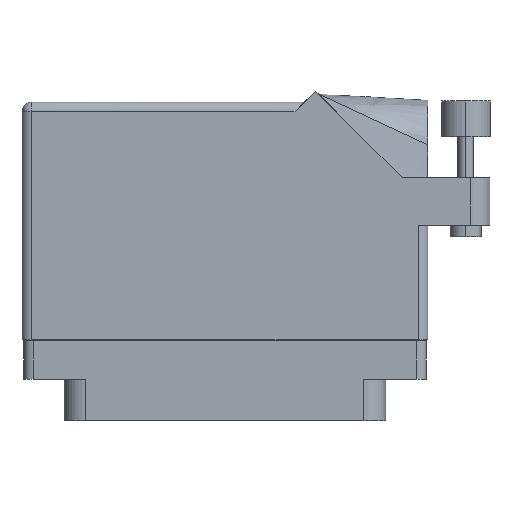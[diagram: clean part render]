
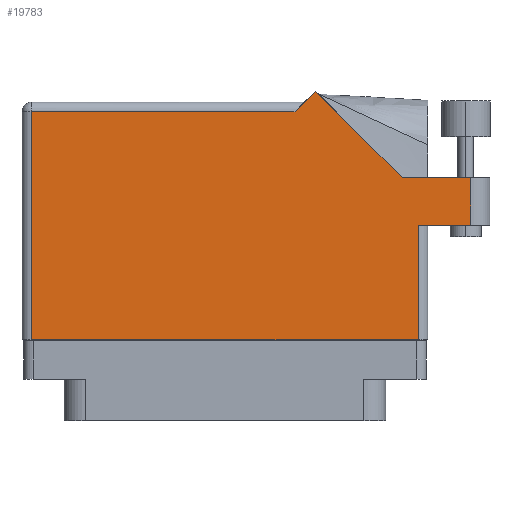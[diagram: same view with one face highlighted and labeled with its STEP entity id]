
A CAD part, front view. The second image highlights one B-rep face of the part: STEP entity #19783.
In plain terms, the highlighted face is planar.
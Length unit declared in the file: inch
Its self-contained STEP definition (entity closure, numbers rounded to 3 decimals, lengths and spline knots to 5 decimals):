
#67 = DIRECTION ( 'NONE',  ( 1., 0., 0. ) ) ;
#538 = LINE ( 'NONE', #2340, #21305 ) ;
#660 = DIRECTION ( 'NONE',  ( -1., 0., 0. ) ) ;
#719 = LINE ( 'NONE', #8086, #8934 ) ;
#1212 = CARTESIAN_POINT ( 'NONE',  ( -1.306, -0.1, 0.455 ) ) ;
#2261 = VERTEX_POINT ( 'NONE', #24734 ) ;
#2340 = CARTESIAN_POINT ( 'NONE',  ( -1.244, -0.1, 0.455 ) ) ;
#3207 = ORIENTED_EDGE ( 'NONE', *, *, #8505, .T. ) ;
#4813 = DIRECTION ( 'NONE',  ( 0., 1., 0. ) ) ;
#5505 = ORIENTED_EDGE ( 'NONE', *, *, #15863, .T. ) ;
#6879 = LINE ( 'NONE', #20447, #30777 ) ;
#7275 = CARTESIAN_POINT ( 'NONE',  ( -1.244, -0.1, 0.455 ) ) ;
#7640 = DIRECTION ( 'NONE',  ( -1., 0., 0. ) ) ;
#8086 = CARTESIAN_POINT ( 'NONE',  ( 1.244, 0.637, 0.455 ) ) ;
#8190 = CARTESIAN_POINT ( 'NONE',  ( 1.306, 0.637, 0.455 ) ) ;
#8468 = CARTESIAN_POINT ( 'NONE',  ( 1.244, 0.637, 0.455 ) ) ;
#8501 = ORIENTED_EDGE ( 'NONE', *, *, #39353, .T. ) ;
#8505 = EDGE_CURVE ( 'NONE', #20362, #31345, #9604, .T. ) ;
#8934 = VECTOR ( 'NONE', #16017, 39.37008 ) ;
#9604 = LINE ( 'NONE', #16311, #18359 ) ;
#9790 = VERTEX_POINT ( 'NONE', #28923 ) ;
#10340 = DIRECTION ( 'NONE',  ( 0., -1., 0. ) ) ;
#10912 = VECTOR ( 'NONE', #50028, 39.37008 ) ;
#11118 = LINE ( 'NONE', #38775, #38047 ) ;
#12791 = EDGE_CURVE ( 'NONE', #9790, #2261, #25380, .T. ) ;
#13012 = CARTESIAN_POINT ( 'NONE',  ( 1.581, 0.637, 0.455 ) ) ;
#13116 = VERTEX_POINT ( 'NONE', #32219 ) ;
#13399 = VECTOR ( 'NONE', #7640, 39.37008 ) ;
#15828 = VECTOR ( 'NONE', #25797, 39.37008 ) ;
#15863 = EDGE_CURVE ( 'NONE', #13116, #21442, #719, .T. ) ;
#16017 = DIRECTION ( 'NONE',  ( 0., 1., 0. ) ) ;
#16311 = CARTESIAN_POINT ( 'NONE',  ( 1.706, 0.944, 0.455 ) ) ;
#16802 = ORIENTED_EDGE ( 'NONE', *, *, #24436, .T. ) ;
#16983 = VECTOR ( 'NONE', #67, 39.37008 ) ;
#18359 = VECTOR ( 'NONE', #48630, 39.37008 ) ;
#18915 = VERTEX_POINT ( 'NONE', #35997 ) ;
#19783 = ADVANCED_FACE ( 'NONE', ( #29522 ), #24737, .F. ) ;
#20362 = VERTEX_POINT ( 'NONE', #50252 ) ;
#20447 = CARTESIAN_POINT ( 'NONE',  ( 1.581, 0.944, 0.455 ) ) ;
#20594 = CARTESIAN_POINT ( 'NONE',  ( 1.14042, 0.944, 0.455 ) ) ;
#20630 = EDGE_CURVE ( 'NONE', #18915, #27556, #538, .T. ) ;
#21305 = VECTOR ( 'NONE', #10340, 39.37008 ) ;
#21442 = VERTEX_POINT ( 'NONE', #8468 ) ;
#22041 = ORIENTED_EDGE ( 'NONE', *, *, #23188, .T. ) ;
#23025 = EDGE_CURVE ( 'NONE', #44366, #20362, #6879, .T. ) ;
#23188 = EDGE_CURVE ( 'NONE', #21442, #44366, #49463, .T. ) ;
#24081 = LINE ( 'NONE', #51544, #13399 ) ;
#24436 = EDGE_CURVE ( 'NONE', #31345, #9790, #11118, .T. ) ;
#24734 = CARTESIAN_POINT ( 'NONE',  ( 0.451, 1.368, 0.455 ) ) ;
#24737 = PLANE ( 'NONE',  #29814 ) ;
#25380 = LINE ( 'NONE', #49537, #10912 ) ;
#25797 = DIRECTION ( 'NONE',  ( 1., 0., 0. ) ) ;
#27556 = VERTEX_POINT ( 'NONE', #7275 ) ;
#28923 = CARTESIAN_POINT ( 'NONE',  ( 0.58371, 1.50071, 0.455 ) ) ;
#29522 = FACE_OUTER_BOUND ( 'NONE', #39858, .T. ) ;
#29814 = AXIS2_PLACEMENT_3D ( 'NONE', #40625, #32978, #660 ) ;
#30777 = VECTOR ( 'NONE', #4813, 39.37008 ) ;
#31345 = VERTEX_POINT ( 'NONE', #20594 ) ;
#32219 = CARTESIAN_POINT ( 'NONE',  ( 1.244, -0.1, 0.455 ) ) ;
#32978 = DIRECTION ( 'NONE',  ( 0., 0., -1. ) ) ;
#35997 = CARTESIAN_POINT ( 'NONE',  ( -1.244, 1.368, 0.455 ) ) ;
#36093 = EDGE_CURVE ( 'NONE', #27556, #13116, #47681, .T. ) ;
#38047 = VECTOR ( 'NONE', #47299, 39.37008 ) ;
#38775 = CARTESIAN_POINT ( 'NONE',  ( 1.14042, 0.944, 0.455 ) ) ;
#39070 = ORIENTED_EDGE ( 'NONE', *, *, #12791, .T. ) ;
#39353 = EDGE_CURVE ( 'NONE', #2261, #18915, #24081, .T. ) ;
#39858 = EDGE_LOOP ( 'NONE', ( #22041, #40624, #3207, #16802, #39070, #8501, #47857, #42623, #5505 ) ) ;
#40624 = ORIENTED_EDGE ( 'NONE', *, *, #23025, .T. ) ;
#40625 = CARTESIAN_POINT ( 'NONE',  ( -1.306, 1.43, 0.455 ) ) ;
#42623 = ORIENTED_EDGE ( 'NONE', *, *, #36093, .T. ) ;
#44366 = VERTEX_POINT ( 'NONE', #13012 ) ;
#47299 = DIRECTION ( 'NONE',  ( -0.707, 0.707, 0. ) ) ;
#47681 = LINE ( 'NONE', #1212, #15828 ) ;
#47857 = ORIENTED_EDGE ( 'NONE', *, *, #20630, .T. ) ;
#48630 = DIRECTION ( 'NONE',  ( -1., 0., 0. ) ) ;
#49463 = LINE ( 'NONE', #8190, #16983 ) ;
#49537 = CARTESIAN_POINT ( 'NONE',  ( 0.513, 1.43, 0.455 ) ) ;
#50028 = DIRECTION ( 'NONE',  ( -0.707, -0.707, 0. ) ) ;
#50252 = CARTESIAN_POINT ( 'NONE',  ( 1.581, 0.944, 0.455 ) ) ;
#51544 = CARTESIAN_POINT ( 'NONE',  ( -1.306, 1.368, 0.455 ) ) ;
